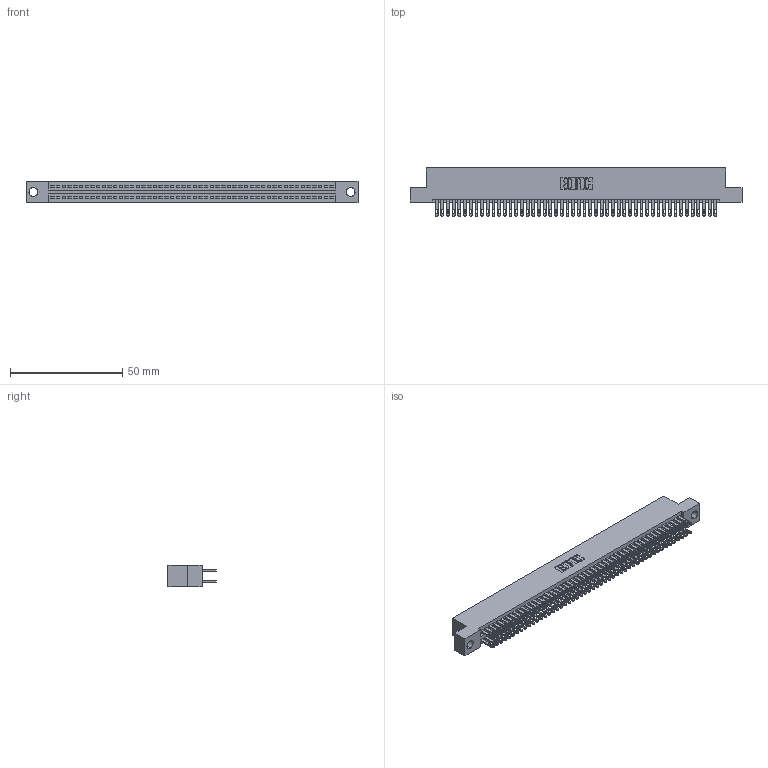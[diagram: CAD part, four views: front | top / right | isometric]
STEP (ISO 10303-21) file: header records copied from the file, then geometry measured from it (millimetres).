
FILE_DESCRIPTION (( 'STEP AP203' ), '1' );
FILE_NAME ('345-100-500-204.STEP', '2018-10-05T12:36:46', ( '' ), ( '' ), 'SwSTEP 2.0', 'SolidWorks 2016', '' );
FILE_SCHEMA (( 'CONFIG_CONTROL_DESIGN' ));
Length unit declared in the file: inch
Products named in the file (3): 345-100-500-204; 345-292-001_345-293-100; 345 Part_Flush Mounting Lugs - 0.156 Dia-TH
Assembly tree (101 placements, depth 2):
  345-100-500-204
    345 Part_Flush Mounting Lugs - 0.156 Dia-TH
    345-292-001_345-293-100  x100
Bounding box: 148.21 x 21.51 x 9.4 mm (x, y, z)
Volume: 14689.2 mm3; surface area: 22703.1 mm2
Topology: 101 solids, 101 shells, 4726 faces, 14441 edges, 9626 vertices
Faces by surface type: plane 2780, cylinder 1946
Entity records: 38087 total; most frequent: CARTESIAN_POINT 6376, ORIENTED_EDGE 6310, DIRECTION 5615, EDGE_CURVE 3155, LINE 2819, VECTOR 2819, VERTEX_POINT 2102, AXIS2_PLACEMENT_3D 1398
